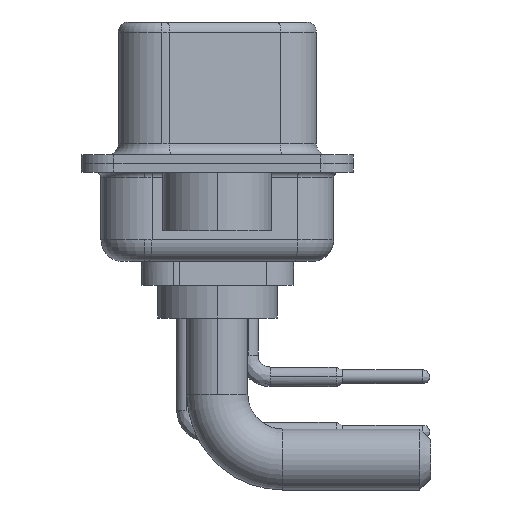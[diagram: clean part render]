
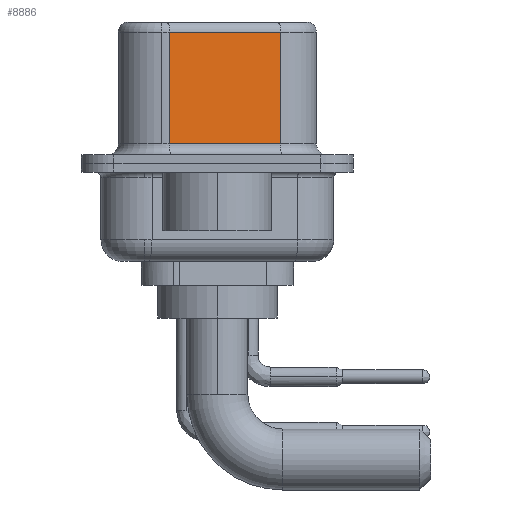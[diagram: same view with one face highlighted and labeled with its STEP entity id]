
A CAD part, left-side view. The second image highlights one B-rep face of the part: STEP entity #8886.
In plain terms, the highlighted planar face has unit normal (-0.985, -0.174, 0).
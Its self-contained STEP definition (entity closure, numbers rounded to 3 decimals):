
#354 = EDGE_CURVE ( 'NONE', #19104, #4644, #13213, .T. ) ;
#683 = CARTESIAN_POINT ( 'NONE',  ( 4.58, -2.897, 6.52 ) ) ;
#2976 = VECTOR ( 'NONE', #5492, 1000. ) ;
#3750 = CARTESIAN_POINT ( 'NONE',  ( 4.58, -2.897, 6.52 ) ) ;
#4268 = VERTEX_POINT ( 'NONE', #6686 ) ;
#4325 = FACE_OUTER_BOUND ( 'NONE', #20251, .T. ) ;
#4390 = AXIS2_PLACEMENT_3D ( 'NONE', #683, #11947, #10194 ) ;
#4644 = VERTEX_POINT ( 'NONE', #21717 ) ;
#5492 = DIRECTION ( 'NONE',  ( -0.174, 0.985, 0. ) ) ;
#6673 = PLANE ( 'NONE',  #4390 ) ;
#6686 = CARTESIAN_POINT ( 'NONE',  ( 4.58, -2.897, 0.9 ) ) ;
#7970 = CARTESIAN_POINT ( 'NONE',  ( 3.68, 2.203, 6.02 ) ) ;
#8007 = DIRECTION ( 'NONE',  ( 0.174, -0.985, 0. ) ) ;
#8886 = ADVANCED_FACE ( 'NONE', ( #4325 ), #6673, .F. ) ;
#9001 = LINE ( 'NONE', #9243, #2976 ) ;
#9243 = CARTESIAN_POINT ( 'NONE',  ( 4.58, -2.897, 6.02 ) ) ;
#10194 = DIRECTION ( 'NONE',  ( -0.174, 0.985, 0. ) ) ;
#10662 = CARTESIAN_POINT ( 'NONE',  ( 4.58, -2.897, 6.02 ) ) ;
#11018 = EDGE_CURVE ( 'NONE', #23516, #4268, #19157, .T. ) ;
#11947 = DIRECTION ( 'NONE',  ( 0.985, 0.174, 0. ) ) ;
#12473 = ORIENTED_EDGE ( 'NONE', *, *, #354, .T. ) ;
#13213 = LINE ( 'NONE', #17334, #17659 ) ;
#15674 = EDGE_CURVE ( 'NONE', #23516, #19104, #9001, .T. ) ;
#16052 = VECTOR ( 'NONE', #22928, 1000. ) ;
#17334 = CARTESIAN_POINT ( 'NONE',  ( 3.68, 2.203, 6.52 ) ) ;
#17645 = LINE ( 'NONE', #21672, #24650 ) ;
#17659 = VECTOR ( 'NONE', #21246, 1000. ) ;
#18571 = ORIENTED_EDGE ( 'NONE', *, *, #20550, .T. ) ;
#19104 = VERTEX_POINT ( 'NONE', #7970 ) ;
#19157 = LINE ( 'NONE', #3750, #16052 ) ;
#19171 = ORIENTED_EDGE ( 'NONE', *, *, #11018, .F. ) ;
#20251 = EDGE_LOOP ( 'NONE', ( #19171, #23852, #12473, #18571 ) ) ;
#20550 = EDGE_CURVE ( 'NONE', #4644, #4268, #17645, .T. ) ;
#21246 = DIRECTION ( 'NONE',  ( 0., 0., -1. ) ) ;
#21672 = CARTESIAN_POINT ( 'NONE',  ( 4.58, -2.897, 0.9 ) ) ;
#21717 = CARTESIAN_POINT ( 'NONE',  ( 3.68, 2.203, 0.9 ) ) ;
#22928 = DIRECTION ( 'NONE',  ( 0., 0., -1. ) ) ;
#23516 = VERTEX_POINT ( 'NONE', #10662 ) ;
#23852 = ORIENTED_EDGE ( 'NONE', *, *, #15674, .T. ) ;
#24650 = VECTOR ( 'NONE', #8007, 1000. ) ;
